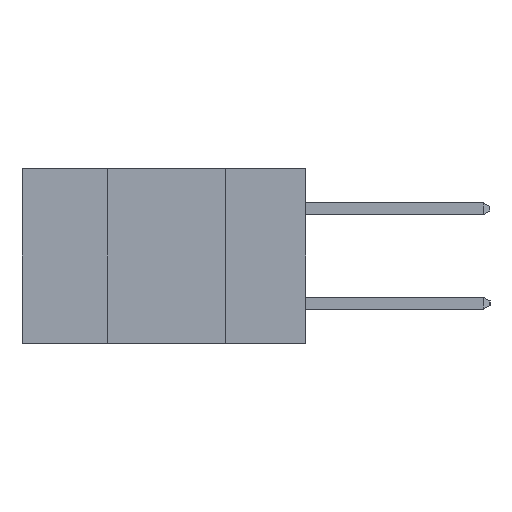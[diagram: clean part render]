
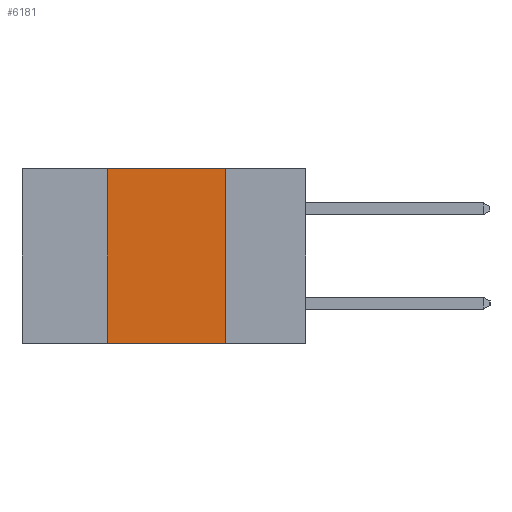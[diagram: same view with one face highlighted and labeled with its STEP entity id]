
A CAD part, left-side view. The second image highlights one B-rep face of the part: STEP entity #6181.
In plain terms, the highlighted planar face has unit normal (-1, 0, 0).
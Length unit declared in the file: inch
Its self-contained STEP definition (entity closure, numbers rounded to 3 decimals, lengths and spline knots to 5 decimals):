
#122 = EDGE_CURVE ( 'NONE', #5398, #12893, #4028, .T. ) ;
#721 = LINE ( 'NONE', #5883, #11844 ) ;
#1662 = VECTOR ( 'NONE', #1921, 39.37008 ) ;
#1765 = CARTESIAN_POINT ( 'NONE',  ( 0., 0.17, -0.37 ) ) ;
#1921 = DIRECTION ( 'NONE',  ( 0., 0., 1. ) ) ;
#2035 = CARTESIAN_POINT ( 'NONE',  ( 0., 0.42, -0.37 ) ) ;
#3738 = VECTOR ( 'NONE', #4029, 39.37008 ) ;
#3994 = CARTESIAN_POINT ( 'NONE',  ( 0., 0.17, -0.37 ) ) ;
#4028 = LINE ( 'NONE', #10748, #12287 ) ;
#4029 = DIRECTION ( 'NONE',  ( 0., 0., -1. ) ) ;
#4732 = EDGE_CURVE ( 'NONE', #11205, #12025, #721, .T. ) ;
#4912 = EDGE_CURVE ( 'NONE', #12893, #12025, #12336, .T. ) ;
#5398 = VERTEX_POINT ( 'NONE', #8235 ) ;
#5428 = ORIENTED_EDGE ( 'NONE', *, *, #6940, .F. ) ;
#5834 = CARTESIAN_POINT ( 'NONE',  ( 0., 0.17, 0. ) ) ;
#5871 = DIRECTION ( 'NONE',  ( 0., -1., 0. ) ) ;
#5883 = CARTESIAN_POINT ( 'NONE',  ( 0., 0.6, -0.37 ) ) ;
#6181 = ADVANCED_FACE ( 'NONE', ( #11124 ), #8603, .F. ) ;
#6720 = AXIS2_PLACEMENT_3D ( 'NONE', #8589, #8555, #8542 ) ;
#6792 = DIRECTION ( 'NONE',  ( 0., -1., 0. ) ) ;
#6940 = EDGE_CURVE ( 'NONE', #11205, #5398, #10271, .T. ) ;
#7124 = ORIENTED_EDGE ( 'NONE', *, *, #122, .F. ) ;
#7248 = CARTESIAN_POINT ( 'NONE',  ( 0., 0.42, -0.37 ) ) ;
#8214 = EDGE_LOOP ( 'NONE', ( #10076, #7124, #5428, #12921 ) ) ;
#8235 = CARTESIAN_POINT ( 'NONE',  ( 0., 0.42, 0. ) ) ;
#8542 = DIRECTION ( 'NONE',  ( 0., 0., -1. ) ) ;
#8555 = DIRECTION ( 'NONE',  ( 1., 0., 0. ) ) ;
#8589 = CARTESIAN_POINT ( 'NONE',  ( 0., 0.6, 0. ) ) ;
#8603 = PLANE ( 'NONE',  #6720 ) ;
#10076 = ORIENTED_EDGE ( 'NONE', *, *, #4912, .F. ) ;
#10271 = LINE ( 'NONE', #2035, #1662 ) ;
#10748 = CARTESIAN_POINT ( 'NONE',  ( 0., 0.6, 0. ) ) ;
#11124 = FACE_OUTER_BOUND ( 'NONE', #8214, .T. ) ;
#11205 = VERTEX_POINT ( 'NONE', #7248 ) ;
#11844 = VECTOR ( 'NONE', #5871, 39.37008 ) ;
#12025 = VERTEX_POINT ( 'NONE', #1765 ) ;
#12287 = VECTOR ( 'NONE', #6792, 39.37008 ) ;
#12336 = LINE ( 'NONE', #3994, #3738 ) ;
#12893 = VERTEX_POINT ( 'NONE', #5834 ) ;
#12921 = ORIENTED_EDGE ( 'NONE', *, *, #4732, .T. ) ;
